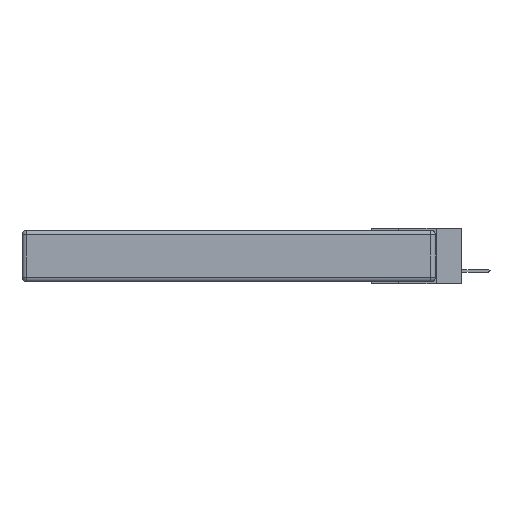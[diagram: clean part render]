
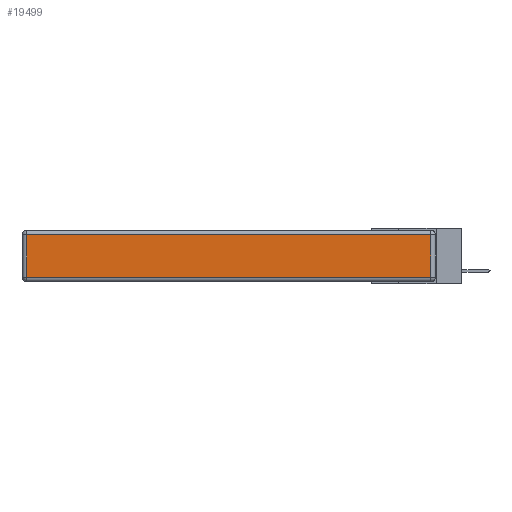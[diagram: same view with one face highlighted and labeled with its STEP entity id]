
A CAD part, left-side view. The second image highlights one B-rep face of the part: STEP entity #19499.
In plain terms, the highlighted planar face has unit normal (-1, 0, 0).
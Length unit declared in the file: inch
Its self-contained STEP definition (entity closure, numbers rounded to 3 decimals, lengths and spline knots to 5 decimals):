
#357 = CARTESIAN_POINT ( 'NONE',  ( 0., 0., -0.313 ) ) ;
#472 = CARTESIAN_POINT ( 'NONE',  ( 0., 2.75, -0.03 ) ) ;
#671 = VERTEX_POINT ( 'NONE', #13615 ) ;
#733 = DIRECTION ( 'NONE',  ( 0., 1., 0. ) ) ;
#1163 = LINE ( 'NONE', #472, #2854 ) ;
#1575 = EDGE_CURVE ( 'NONE', #7654, #671, #6793, .T. ) ;
#2854 = VECTOR ( 'NONE', #733, 39.37008 ) ;
#3156 = VECTOR ( 'NONE', #16615, 39.37008 ) ;
#3239 = VECTOR ( 'NONE', #9103, 39.37008 ) ;
#3556 = DIRECTION ( 'NONE',  ( 0., -1., 0. ) ) ;
#4181 = FACE_OUTER_BOUND ( 'NONE', #8802, .T. ) ;
#4363 = CARTESIAN_POINT ( 'NONE',  ( 0., 2.72, -0.343 ) ) ;
#4539 = AXIS2_PLACEMENT_3D ( 'NONE', #12559, #8139, #10980 ) ;
#5331 = VECTOR ( 'NONE', #3556, 39.37008 ) ;
#6316 = EDGE_CURVE ( 'NONE', #671, #8866, #1163, .T. ) ;
#6793 = LINE ( 'NONE', #11860, #3156 ) ;
#7654 = VERTEX_POINT ( 'NONE', #19193 ) ;
#8139 = DIRECTION ( 'NONE',  ( -1., 0., 0. ) ) ;
#8802 = EDGE_LOOP ( 'NONE', ( #18035, #14764, #9812, #19684 ) ) ;
#8866 = VERTEX_POINT ( 'NONE', #9136 ) ;
#9103 = DIRECTION ( 'NONE',  ( 0., 0., -1. ) ) ;
#9136 = CARTESIAN_POINT ( 'NONE',  ( 0., 2.72, -0.03 ) ) ;
#9398 = EDGE_CURVE ( 'NONE', #8866, #14850, #9480, .T. ) ;
#9480 = LINE ( 'NONE', #4363, #3239 ) ;
#9497 = PLANE ( 'NONE',  #4539 ) ;
#9812 = ORIENTED_EDGE ( 'NONE', *, *, #6316, .T. ) ;
#10980 = DIRECTION ( 'NONE',  ( 0., 0., 1. ) ) ;
#11860 = CARTESIAN_POINT ( 'NONE',  ( 0., 0.03, -0.343 ) ) ;
#12559 = CARTESIAN_POINT ( 'NONE',  ( 0., 0., -0.343 ) ) ;
#13615 = CARTESIAN_POINT ( 'NONE',  ( 0., 0.03, -0.03 ) ) ;
#13984 = EDGE_CURVE ( 'NONE', #14850, #7654, #14757, .T. ) ;
#14757 = LINE ( 'NONE', #357, #5331 ) ;
#14764 = ORIENTED_EDGE ( 'NONE', *, *, #1575, .T. ) ;
#14850 = VERTEX_POINT ( 'NONE', #19385 ) ;
#16615 = DIRECTION ( 'NONE',  ( 0., 0., 1. ) ) ;
#18035 = ORIENTED_EDGE ( 'NONE', *, *, #13984, .T. ) ;
#19193 = CARTESIAN_POINT ( 'NONE',  ( 0., 0.03, -0.313 ) ) ;
#19385 = CARTESIAN_POINT ( 'NONE',  ( 0., 2.72, -0.313 ) ) ;
#19499 = ADVANCED_FACE ( 'NONE', ( #4181 ), #9497, .T. ) ;
#19684 = ORIENTED_EDGE ( 'NONE', *, *, #9398, .T. ) ;
